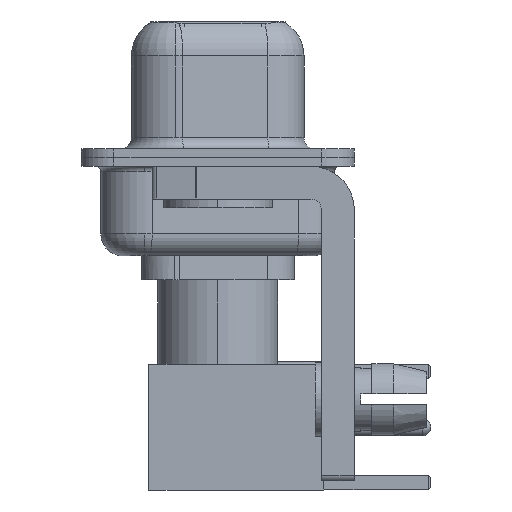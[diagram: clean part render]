
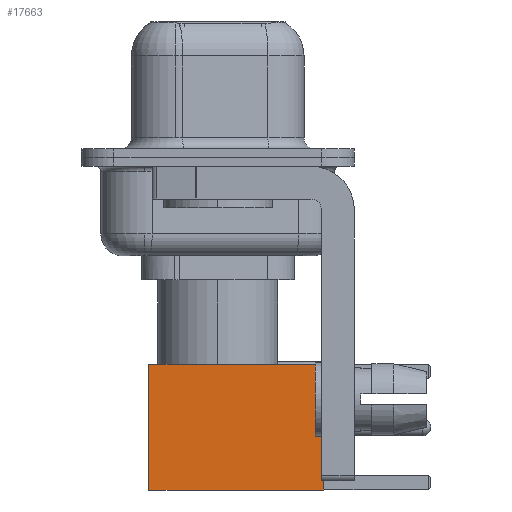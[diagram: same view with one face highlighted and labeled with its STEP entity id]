
A CAD part, left-side view. The second image highlights one B-rep face of the part: STEP entity #17663.
In plain terms, the highlighted face is planar.
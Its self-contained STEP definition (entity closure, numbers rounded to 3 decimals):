
#608 = EDGE_CURVE ( 'NONE', #16859, #8874, #1817, .T. ) ;
#826 = VECTOR ( 'NONE', #4111, 1000. ) ;
#1817 = LINE ( 'NONE', #18116, #826 ) ;
#2286 = VECTOR ( 'NONE', #23275, 1000. ) ;
#3634 = CARTESIAN_POINT ( 'NONE',  ( -2.875, 2.875, 8. ) ) ;
#4111 = DIRECTION ( 'NONE',  ( -1., 0., 0. ) ) ;
#8322 = ORIENTED_EDGE ( 'NONE', *, *, #608, .F. ) ;
#8874 = VERTEX_POINT ( 'NONE', #3634 ) ;
#9860 = DIRECTION ( 'NONE',  ( 0., 0., 1. ) ) ;
#10209 = LINE ( 'NONE', #14526, #15666 ) ;
#10525 = DIRECTION ( 'NONE',  ( 0., 0., -1. ) ) ;
#12359 = VECTOR ( 'NONE', #10525, 1000. ) ;
#13707 = CARTESIAN_POINT ( 'NONE',  ( 2.875, 2.875, 0. ) ) ;
#13882 = DIRECTION ( 'NONE',  ( 0., 1., 0. ) ) ;
#13899 = LINE ( 'NONE', #23409, #2286 ) ;
#14201 = EDGE_CURVE ( 'NONE', #8874, #17281, #22935, .T. ) ;
#14249 = CARTESIAN_POINT ( 'NONE',  ( 2.875, 2.875, 8. ) ) ;
#14526 = CARTESIAN_POINT ( 'NONE',  ( 0., 2.875, 0. ) ) ;
#15081 = ORIENTED_EDGE ( 'NONE', *, *, #14201, .F. ) ;
#15666 = VECTOR ( 'NONE', #16013, 1000. ) ;
#16013 = DIRECTION ( 'NONE',  ( -1., 0., 0. ) ) ;
#16323 = CARTESIAN_POINT ( 'NONE',  ( -2.875, 2.875, 0. ) ) ;
#16859 = VERTEX_POINT ( 'NONE', #14249 ) ;
#17281 = VERTEX_POINT ( 'NONE', #17460 ) ;
#17460 = CARTESIAN_POINT ( 'NONE',  ( -2.875, 2.875, 0. ) ) ;
#17663 = ADVANCED_FACE ( 'NONE', ( #21849 ), #17803, .T. ) ;
#17803 = PLANE ( 'NONE',  #25375 ) ;
#18116 = CARTESIAN_POINT ( 'NONE',  ( 0., 2.875, 8. ) ) ;
#18451 = VERTEX_POINT ( 'NONE', #13707 ) ;
#21639 = EDGE_LOOP ( 'NONE', ( #24960, #21647, #15081, #8322 ) ) ;
#21647 = ORIENTED_EDGE ( 'NONE', *, *, #25455, .T. ) ;
#21849 = FACE_OUTER_BOUND ( 'NONE', #21639, .T. ) ;
#22935 = LINE ( 'NONE', #16323, #12359 ) ;
#23042 = EDGE_CURVE ( 'NONE', #16859, #18451, #13899, .T. ) ;
#23275 = DIRECTION ( 'NONE',  ( 0., 0., -1. ) ) ;
#23409 = CARTESIAN_POINT ( 'NONE',  ( 2.875, 2.875, 0. ) ) ;
#24960 = ORIENTED_EDGE ( 'NONE', *, *, #23042, .T. ) ;
#25375 = AXIS2_PLACEMENT_3D ( 'NONE', #26318, #13882, #9860 ) ;
#25455 = EDGE_CURVE ( 'NONE', #18451, #17281, #10209, .T. ) ;
#26318 = CARTESIAN_POINT ( 'NONE',  ( 2.875, 2.875, 0. ) ) ;
